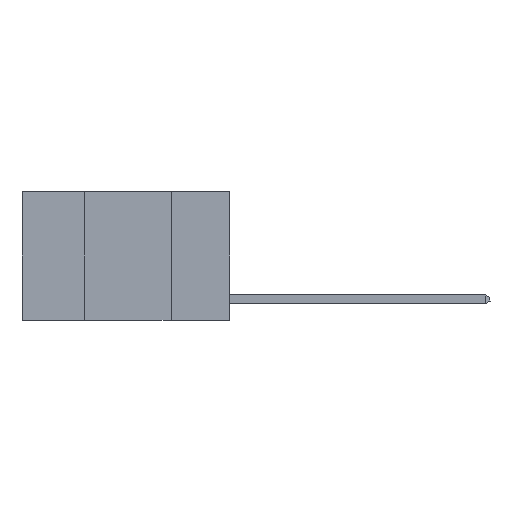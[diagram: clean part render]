
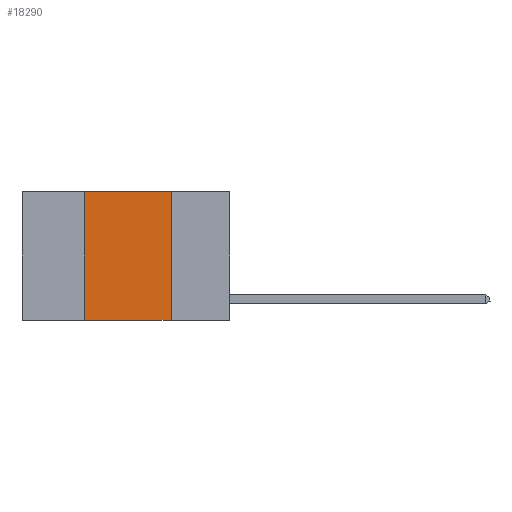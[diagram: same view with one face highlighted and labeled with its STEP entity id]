
A CAD part, left-side view. The second image highlights one B-rep face of the part: STEP entity #18290.
In plain terms, the highlighted planar face has unit normal (-1, 0, 0).
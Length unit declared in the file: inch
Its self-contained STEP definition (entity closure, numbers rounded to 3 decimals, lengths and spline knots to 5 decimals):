
#1690 = VECTOR ( 'NONE', #22573, 39.37008 ) ;
#2058 = VECTOR ( 'NONE', #23250, 39.37008 ) ;
#2768 = VERTEX_POINT ( 'NONE', #26872 ) ;
#4293 = CARTESIAN_POINT ( 'NONE',  ( 0., 0.6, 0. ) ) ;
#6158 = CARTESIAN_POINT ( 'NONE',  ( 0., 0.17, -0.37 ) ) ;
#7209 = EDGE_LOOP ( 'NONE', ( #25174, #16609, #21631, #14367 ) ) ;
#9329 = VERTEX_POINT ( 'NONE', #23035 ) ;
#9878 = CARTESIAN_POINT ( 'NONE',  ( 0., 0.6, -0.37 ) ) ;
#11136 = DIRECTION ( 'NONE',  ( 1., 0., 0. ) ) ;
#11448 = CARTESIAN_POINT ( 'NONE',  ( 0., 0.6, 0. ) ) ;
#13848 = LINE ( 'NONE', #11448, #1690 ) ;
#14367 = ORIENTED_EDGE ( 'NONE', *, *, #27624, .T. ) ;
#16419 = CARTESIAN_POINT ( 'NONE',  ( 0., 0.42, -0.37 ) ) ;
#16609 = ORIENTED_EDGE ( 'NONE', *, *, #27433, .F. ) ;
#17616 = CARTESIAN_POINT ( 'NONE',  ( 0., 0.42, 0. ) ) ;
#18046 = FACE_OUTER_BOUND ( 'NONE', #7209, .T. ) ;
#18290 = ADVANCED_FACE ( 'NONE', ( #18046 ), #24511, .F. ) ;
#18740 = EDGE_CURVE ( 'NONE', #2768, #28504, #29042, .T. ) ;
#20083 = LINE ( 'NONE', #9878, #2058 ) ;
#20242 = AXIS2_PLACEMENT_3D ( 'NONE', #4293, #11136, #26692 ) ;
#20337 = VECTOR ( 'NONE', #26541, 39.37008 ) ;
#20644 = VERTEX_POINT ( 'NONE', #16419 ) ;
#21631 = ORIENTED_EDGE ( 'NONE', *, *, #29074, .F. ) ;
#22573 = DIRECTION ( 'NONE',  ( 0., -1., 0. ) ) ;
#23035 = CARTESIAN_POINT ( 'NONE',  ( 0., 0.42, 0. ) ) ;
#23246 = VECTOR ( 'NONE', #25563, 39.37008 ) ;
#23250 = DIRECTION ( 'NONE',  ( 0., -1., 0. ) ) ;
#23341 = CARTESIAN_POINT ( 'NONE',  ( 0., 0.17, 0. ) ) ;
#24511 = PLANE ( 'NONE',  #20242 ) ;
#25174 = ORIENTED_EDGE ( 'NONE', *, *, #18740, .F. ) ;
#25563 = DIRECTION ( 'NONE',  ( 0., 0., -1. ) ) ;
#26264 = LINE ( 'NONE', #17616, #20337 ) ;
#26541 = DIRECTION ( 'NONE',  ( 0., 0., 1. ) ) ;
#26692 = DIRECTION ( 'NONE',  ( 0., 0., -1. ) ) ;
#26872 = CARTESIAN_POINT ( 'NONE',  ( 0., 0.17, 0. ) ) ;
#27433 = EDGE_CURVE ( 'NONE', #9329, #2768, #13848, .T. ) ;
#27624 = EDGE_CURVE ( 'NONE', #20644, #28504, #20083, .T. ) ;
#28504 = VERTEX_POINT ( 'NONE', #6158 ) ;
#29042 = LINE ( 'NONE', #23341, #23246 ) ;
#29074 = EDGE_CURVE ( 'NONE', #20644, #9329, #26264, .T. ) ;
